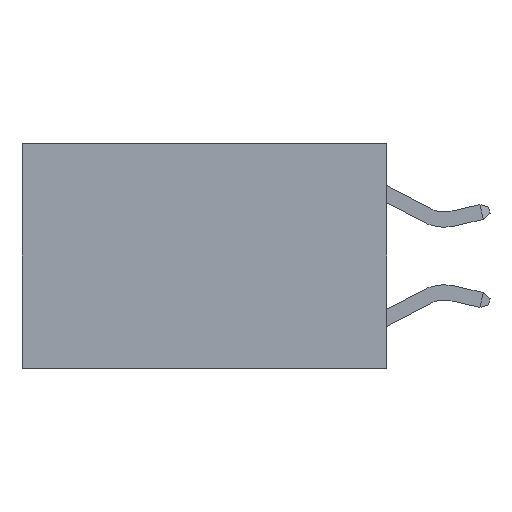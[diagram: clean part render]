
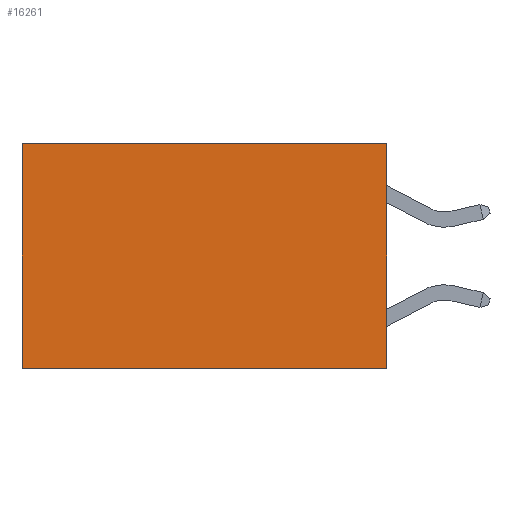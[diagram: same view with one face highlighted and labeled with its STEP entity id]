
A CAD part, left-side view. The second image highlights one B-rep face of the part: STEP entity #16261.
In plain terms, the highlighted planar face has unit normal (-1, 0, 0).
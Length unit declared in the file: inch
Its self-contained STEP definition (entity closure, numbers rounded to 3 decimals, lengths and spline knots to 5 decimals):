
#57 = EDGE_CURVE ( 'NONE', #6126, #14714, #5270, .T. ) ;
#522 = VERTEX_POINT ( 'NONE', #11056 ) ;
#564 = CARTESIAN_POINT ( 'NONE',  ( 0.2625, 0., 0. ) ) ;
#918 = DIRECTION ( 'NONE',  ( 0., 0., -1. ) ) ;
#3173 = ORIENTED_EDGE ( 'NONE', *, *, #57, .T. ) ;
#3341 = CARTESIAN_POINT ( 'NONE',  ( 0.2625, 0., -0.37 ) ) ;
#3651 = AXIS2_PLACEMENT_3D ( 'NONE', #3828, #5145, #918 ) ;
#3828 = CARTESIAN_POINT ( 'NONE',  ( 0.2625, 0., 0. ) ) ;
#3877 = FACE_OUTER_BOUND ( 'NONE', #7532, .T. ) ;
#5145 = DIRECTION ( 'NONE',  ( 1., 0., 0. ) ) ;
#5270 = LINE ( 'NONE', #17199, #7272 ) ;
#6113 = EDGE_CURVE ( 'NONE', #6126, #14304, #14859, .T. ) ;
#6126 = VERTEX_POINT ( 'NONE', #564 ) ;
#6219 = DIRECTION ( 'NONE',  ( 0., 0., -1. ) ) ;
#7272 = VECTOR ( 'NONE', #10102, 39.37008 ) ;
#7532 = EDGE_LOOP ( 'NONE', ( #13789, #17435, #15633, #3173 ) ) ;
#8523 = EDGE_CURVE ( 'NONE', #14304, #522, #16317, .T. ) ;
#9262 = EDGE_CURVE ( 'NONE', #14714, #522, #13094, .T. ) ;
#9591 = DIRECTION ( 'NONE',  ( 0., 1., 0. ) ) ;
#10102 = DIRECTION ( 'NONE',  ( 0., 1., 0. ) ) ;
#11027 = VECTOR ( 'NONE', #6219, 39.37008 ) ;
#11056 = CARTESIAN_POINT ( 'NONE',  ( 0.2625, 0.6, -0.37 ) ) ;
#12391 = PLANE ( 'NONE',  #3651 ) ;
#13094 = LINE ( 'NONE', #15735, #17188 ) ;
#13423 = CARTESIAN_POINT ( 'NONE',  ( 0.2625, 0., 0. ) ) ;
#13789 = ORIENTED_EDGE ( 'NONE', *, *, #9262, .T. ) ;
#14304 = VERTEX_POINT ( 'NONE', #3341 ) ;
#14714 = VERTEX_POINT ( 'NONE', #16382 ) ;
#14859 = LINE ( 'NONE', #13423, #11027 ) ;
#15405 = CARTESIAN_POINT ( 'NONE',  ( 0.2625, 0., -0.37 ) ) ;
#15540 = DIRECTION ( 'NONE',  ( 0., 0., -1. ) ) ;
#15622 = VECTOR ( 'NONE', #9591, 39.37008 ) ;
#15633 = ORIENTED_EDGE ( 'NONE', *, *, #6113, .F. ) ;
#15735 = CARTESIAN_POINT ( 'NONE',  ( 0.2625, 0.6, 0. ) ) ;
#16261 = ADVANCED_FACE ( 'NONE', ( #3877 ), #12391, .F. ) ;
#16317 = LINE ( 'NONE', #15405, #15622 ) ;
#16382 = CARTESIAN_POINT ( 'NONE',  ( 0.2625, 0.6, 0. ) ) ;
#17188 = VECTOR ( 'NONE', #15540, 39.37008 ) ;
#17199 = CARTESIAN_POINT ( 'NONE',  ( 0.2625, 0., 0. ) ) ;
#17435 = ORIENTED_EDGE ( 'NONE', *, *, #8523, .F. ) ;
